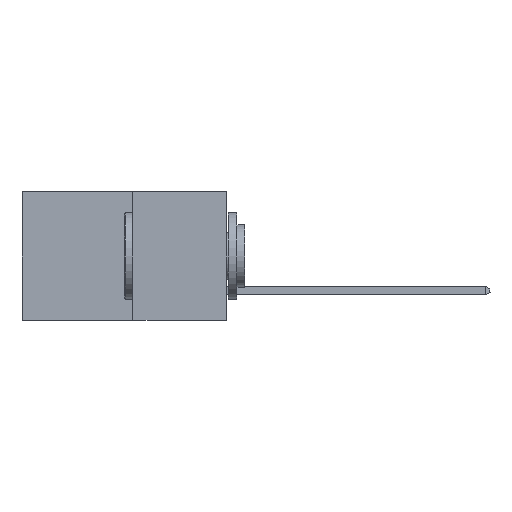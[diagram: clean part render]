
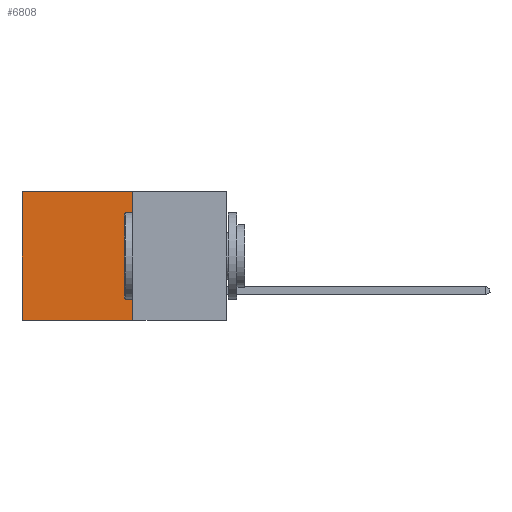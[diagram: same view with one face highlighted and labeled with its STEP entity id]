
A CAD part, left-side view. The second image highlights one B-rep face of the part: STEP entity #6808.
In plain terms, the highlighted planar face has unit normal (-1, 0, 0).
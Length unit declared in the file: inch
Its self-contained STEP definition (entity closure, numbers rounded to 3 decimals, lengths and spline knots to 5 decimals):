
#578 = ORIENTED_EDGE ( 'NONE', *, *, #7310, .T. ) ;
#856 = ORIENTED_EDGE ( 'NONE', *, *, #13728, .T. ) ;
#1839 = AXIS2_PLACEMENT_3D ( 'NONE', #4150, #4125, #4102 ) ;
#1919 = EDGE_CURVE ( 'NONE', #4142, #2766, #12494, .T. ) ;
#2687 = CARTESIAN_POINT ( 'NONE',  ( 0.277, 0.59, -0.37 ) ) ;
#2766 = VERTEX_POINT ( 'NONE', #16017 ) ;
#2805 = VERTEX_POINT ( 'NONE', #2687 ) ;
#3400 = CARTESIAN_POINT ( 'NONE',  ( 0.277, 0.59, 0. ) ) ;
#4102 = DIRECTION ( 'NONE',  ( 0., 0., -1. ) ) ;
#4125 = DIRECTION ( 'NONE',  ( 1., 0., 0. ) ) ;
#4142 = VERTEX_POINT ( 'NONE', #21928 ) ;
#4150 = CARTESIAN_POINT ( 'NONE',  ( 0.277, 0.27, -0.37 ) ) ;
#4183 = PLANE ( 'NONE',  #1839 ) ;
#4283 = LINE ( 'NONE', #7890, #17266 ) ;
#6297 = EDGE_LOOP ( 'NONE', ( #856, #14978, #13306, #578 ) ) ;
#6808 = ADVANCED_FACE ( 'NONE', ( #10815 ), #4183, .F. ) ;
#7310 = EDGE_CURVE ( 'NONE', #4142, #16261, #14530, .T. ) ;
#7566 = VECTOR ( 'NONE', #21986, 39.37008 ) ;
#7890 = CARTESIAN_POINT ( 'NONE',  ( 0.277, 0.27, -0.37 ) ) ;
#8407 = VECTOR ( 'NONE', #16428, 39.37008 ) ;
#8988 = LINE ( 'NONE', #10892, #8407 ) ;
#10815 = FACE_OUTER_BOUND ( 'NONE', #6297, .T. ) ;
#10892 = CARTESIAN_POINT ( 'NONE',  ( 0.277, 0.59, -0.37 ) ) ;
#12494 = LINE ( 'NONE', #21222, #7566 ) ;
#13306 = ORIENTED_EDGE ( 'NONE', *, *, #1919, .F. ) ;
#13728 = EDGE_CURVE ( 'NONE', #16261, #2805, #8988, .T. ) ;
#13977 = EDGE_CURVE ( 'NONE', #2766, #2805, #4283, .T. ) ;
#14530 = LINE ( 'NONE', #18654, #23498 ) ;
#14978 = ORIENTED_EDGE ( 'NONE', *, *, #13977, .F. ) ;
#16017 = CARTESIAN_POINT ( 'NONE',  ( 0.277, 0.27, -0.37 ) ) ;
#16261 = VERTEX_POINT ( 'NONE', #3400 ) ;
#16428 = DIRECTION ( 'NONE',  ( 0., 0., -1. ) ) ;
#17266 = VECTOR ( 'NONE', #20682, 39.37008 ) ;
#18054 = DIRECTION ( 'NONE',  ( 0., 1., 0. ) ) ;
#18654 = CARTESIAN_POINT ( 'NONE',  ( 0.277, 0.27, 0. ) ) ;
#20682 = DIRECTION ( 'NONE',  ( 0., 1., 0. ) ) ;
#21222 = CARTESIAN_POINT ( 'NONE',  ( 0.277, 0.27, -0.37 ) ) ;
#21928 = CARTESIAN_POINT ( 'NONE',  ( 0.277, 0.27, 0. ) ) ;
#21986 = DIRECTION ( 'NONE',  ( 0., 0., -1. ) ) ;
#23498 = VECTOR ( 'NONE', #18054, 39.37008 ) ;
